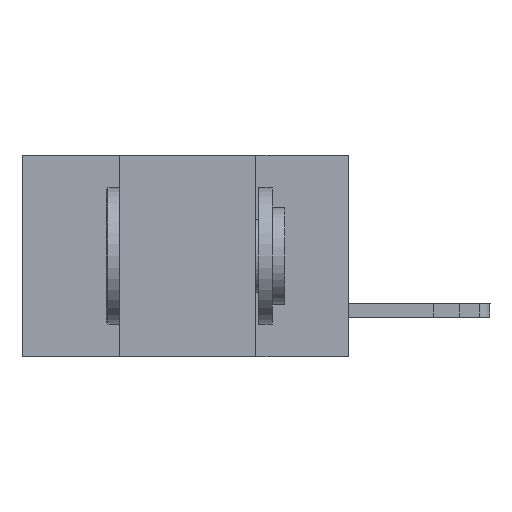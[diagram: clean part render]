
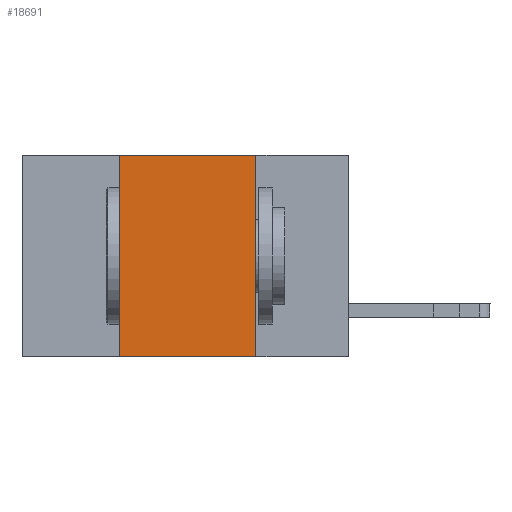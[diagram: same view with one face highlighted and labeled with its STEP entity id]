
A CAD part, left-side view. The second image highlights one B-rep face of the part: STEP entity #18691.
In plain terms, the highlighted planar face has unit normal (-1, 0, 0).
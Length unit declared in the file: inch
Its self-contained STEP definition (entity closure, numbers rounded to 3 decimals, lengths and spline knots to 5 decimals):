
#34 = VECTOR ( 'NONE', #17262, 39.37008 ) ;
#338 = CARTESIAN_POINT ( 'NONE',  ( 0., 0.6, -0.37 ) ) ;
#605 = VERTEX_POINT ( 'NONE', #3601 ) ;
#1179 = VECTOR ( 'NONE', #7262, 39.37008 ) ;
#1537 = ORIENTED_EDGE ( 'NONE', *, *, #6427, .F. ) ;
#2035 = EDGE_CURVE ( 'NONE', #15529, #7003, #4403, .T. ) ;
#2220 = ORIENTED_EDGE ( 'NONE', *, *, #5993, .F. ) ;
#3120 = ORIENTED_EDGE ( 'NONE', *, *, #2035, .F. ) ;
#3601 = CARTESIAN_POINT ( 'NONE',  ( 0., 0.17, 0. ) ) ;
#3713 = DIRECTION ( 'NONE',  ( 0., 0., -1. ) ) ;
#4302 = CARTESIAN_POINT ( 'NONE',  ( 0., 0.42, -0.37 ) ) ;
#4403 = LINE ( 'NONE', #4302, #19821 ) ;
#5993 = EDGE_CURVE ( 'NONE', #605, #7199, #12161, .T. ) ;
#6427 = EDGE_CURVE ( 'NONE', #7003, #605, #8778, .T. ) ;
#7003 = VERTEX_POINT ( 'NONE', #8449 ) ;
#7199 = VERTEX_POINT ( 'NONE', #13524 ) ;
#7262 = DIRECTION ( 'NONE',  ( 0., 0., -1. ) ) ;
#7780 = LINE ( 'NONE', #338, #34 ) ;
#8402 = FACE_OUTER_BOUND ( 'NONE', #18601, .T. ) ;
#8449 = CARTESIAN_POINT ( 'NONE',  ( 0., 0.42, 0. ) ) ;
#8778 = LINE ( 'NONE', #19799, #15465 ) ;
#9109 = DIRECTION ( 'NONE',  ( 0., 0., 1. ) ) ;
#12161 = LINE ( 'NONE', #14912, #1179 ) ;
#13383 = EDGE_CURVE ( 'NONE', #15529, #7199, #7780, .T. ) ;
#13524 = CARTESIAN_POINT ( 'NONE',  ( 0., 0.17, -0.37 ) ) ;
#14608 = CARTESIAN_POINT ( 'NONE',  ( 0., 0.6, 0. ) ) ;
#14912 = CARTESIAN_POINT ( 'NONE',  ( 0., 0.17, -0.37 ) ) ;
#15465 = VECTOR ( 'NONE', #19597, 39.37008 ) ;
#15529 = VERTEX_POINT ( 'NONE', #15637 ) ;
#15637 = CARTESIAN_POINT ( 'NONE',  ( 0., 0.42, -0.37 ) ) ;
#17162 = ORIENTED_EDGE ( 'NONE', *, *, #13383, .T. ) ;
#17262 = DIRECTION ( 'NONE',  ( 0., -1., 0. ) ) ;
#17481 = DIRECTION ( 'NONE',  ( 1., 0., 0. ) ) ;
#17684 = PLANE ( 'NONE',  #19025 ) ;
#18601 = EDGE_LOOP ( 'NONE', ( #2220, #1537, #3120, #17162 ) ) ;
#18691 = ADVANCED_FACE ( 'NONE', ( #8402 ), #17684, .F. ) ;
#19025 = AXIS2_PLACEMENT_3D ( 'NONE', #14608, #17481, #3713 ) ;
#19597 = DIRECTION ( 'NONE',  ( 0., -1., 0. ) ) ;
#19799 = CARTESIAN_POINT ( 'NONE',  ( 0., 0.6, 0. ) ) ;
#19821 = VECTOR ( 'NONE', #9109, 39.37008 ) ;
